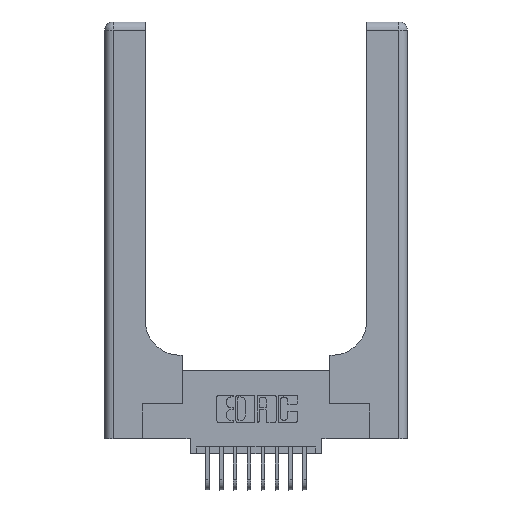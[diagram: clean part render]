
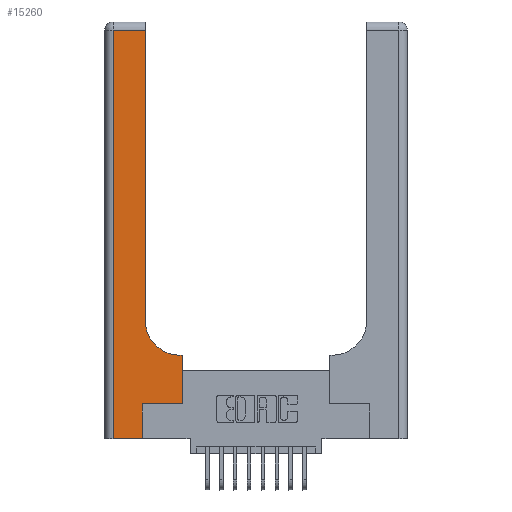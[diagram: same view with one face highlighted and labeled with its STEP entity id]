
A CAD part, top view. The second image highlights one B-rep face of the part: STEP entity #15260.
In plain terms, the highlighted planar face has unit normal (0, 0, 1).
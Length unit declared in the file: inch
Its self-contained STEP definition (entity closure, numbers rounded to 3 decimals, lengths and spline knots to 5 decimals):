
#75 = LINE ( 'NONE', #4057, #527 ) ;
#527 = VECTOR ( 'NONE', #12384, 39.37008 ) ;
#1086 = CARTESIAN_POINT ( 'NONE',  ( 0.2915, 2.94, 0.37 ) ) ;
#1235 = CARTESIAN_POINT ( 'NONE',  ( 0.2915, 0.6, 0.37 ) ) ;
#1479 = PLANE ( 'NONE',  #1958 ) ;
#1505 = CARTESIAN_POINT ( 'NONE',  ( 0.5415, 0.6, 0.37 ) ) ;
#1958 = AXIS2_PLACEMENT_3D ( 'NONE', #9866, #2883, #12638 ) ;
#2146 = CARTESIAN_POINT ( 'NONE',  ( 0.2915, 3., 0.37 ) ) ;
#2155 = VECTOR ( 'NONE', #7720, 39.37008 ) ;
#2588 = LINE ( 'NONE', #2146, #2155 ) ;
#2624 = CARTESIAN_POINT ( 'NONE',  ( 0.269, 0., 0.37 ) ) ;
#2649 = DIRECTION ( 'NONE',  ( -1., 0., 0. ) ) ;
#2883 = DIRECTION ( 'NONE',  ( 0., 0., -1. ) ) ;
#3165 = LINE ( 'NONE', #17815, #17306 ) ;
#3261 = VERTEX_POINT ( 'NONE', #2624 ) ;
#3745 = LINE ( 'NONE', #1235, #10744 ) ;
#3782 = ORIENTED_EDGE ( 'NONE', *, *, #10803, .T. ) ;
#3843 = EDGE_CURVE ( 'NONE', #6789, #8115, #2588, .T. ) ;
#4057 = CARTESIAN_POINT ( 'NONE',  ( 0.269, 0.25, 0.37 ) ) ;
#4095 = ORIENTED_EDGE ( 'NONE', *, *, #15156, .T. ) ;
#4213 = VECTOR ( 'NONE', #13894, 39.37008 ) ;
#4216 = VERTEX_POINT ( 'NONE', #5692 ) ;
#4262 = ORIENTED_EDGE ( 'NONE', *, *, #5912, .T. ) ;
#4640 = LINE ( 'NONE', #13652, #15166 ) ;
#4658 = LINE ( 'NONE', #5615, #4213 ) ;
#5382 = CIRCLE ( 'NONE', #16242, 0.25 ) ;
#5615 = CARTESIAN_POINT ( 'NONE',  ( 0.06, 3., 0.37 ) ) ;
#5692 = CARTESIAN_POINT ( 'NONE',  ( 0.06, 0., 0.37 ) ) ;
#5752 = CARTESIAN_POINT ( 'NONE',  ( 0.5415, 0.85, 0.37 ) ) ;
#5762 = EDGE_CURVE ( 'NONE', #10571, #16123, #75, .T. ) ;
#5819 = VECTOR ( 'NONE', #16554, 39.37008 ) ;
#5849 = EDGE_CURVE ( 'NONE', #4216, #3261, #11697, .T. ) ;
#5912 = EDGE_CURVE ( 'NONE', #14706, #6789, #5382, .T. ) ;
#6471 = EDGE_CURVE ( 'NONE', #8115, #14822, #3165, .T. ) ;
#6789 = VERTEX_POINT ( 'NONE', #10384 ) ;
#6978 = ORIENTED_EDGE ( 'NONE', *, *, #3843, .T. ) ;
#7153 = DIRECTION ( 'NONE',  ( 1., 0., 0. ) ) ;
#7691 = ORIENTED_EDGE ( 'NONE', *, *, #14671, .T. ) ;
#7720 = DIRECTION ( 'NONE',  ( 0., 1., 0. ) ) ;
#7810 = VECTOR ( 'NONE', #10729, 39.37008 ) ;
#8115 = VERTEX_POINT ( 'NONE', #1086 ) ;
#8242 = LINE ( 'NONE', #17394, #7810 ) ;
#8479 = VERTEX_POINT ( 'NONE', #12907 ) ;
#8580 = ORIENTED_EDGE ( 'NONE', *, *, #5762, .T. ) ;
#8990 = FACE_OUTER_BOUND ( 'NONE', #13356, .T. ) ;
#9780 = DIRECTION ( 'NONE',  ( -1., 0., 0. ) ) ;
#9866 = CARTESIAN_POINT ( 'NONE',  ( 0., 3., 0.37 ) ) ;
#10266 = CARTESIAN_POINT ( 'NONE',  ( 0.06, 2.94, 0.37 ) ) ;
#10384 = CARTESIAN_POINT ( 'NONE',  ( 0.2915, 0.85, 0.37 ) ) ;
#10571 = VERTEX_POINT ( 'NONE', #15611 ) ;
#10729 = DIRECTION ( 'NONE',  ( 0., 1., 0. ) ) ;
#10744 = VECTOR ( 'NONE', #2649, 39.37008 ) ;
#10803 = EDGE_CURVE ( 'NONE', #16123, #8479, #8242, .T. ) ;
#11697 = LINE ( 'NONE', #17825, #5819 ) ;
#12384 = DIRECTION ( 'NONE',  ( 1., 0., 0. ) ) ;
#12638 = DIRECTION ( 'NONE',  ( -1., 0., 0. ) ) ;
#12907 = CARTESIAN_POINT ( 'NONE',  ( 0.5585, 0.6, 0.37 ) ) ;
#13356 = EDGE_LOOP ( 'NONE', ( #6978, #17021, #7691, #13748, #15027, #8580, #3782, #4095, #4262 ) ) ;
#13652 = CARTESIAN_POINT ( 'NONE',  ( 0.269, 0., 0.37 ) ) ;
#13748 = ORIENTED_EDGE ( 'NONE', *, *, #5849, .T. ) ;
#13794 = CARTESIAN_POINT ( 'NONE',  ( 0.5585, 0.25, 0.37 ) ) ;
#13894 = DIRECTION ( 'NONE',  ( 0., -1., 0. ) ) ;
#14671 = EDGE_CURVE ( 'NONE', #14822, #4216, #4658, .T. ) ;
#14706 = VERTEX_POINT ( 'NONE', #1505 ) ;
#14822 = VERTEX_POINT ( 'NONE', #10266 ) ;
#15027 = ORIENTED_EDGE ( 'NONE', *, *, #15102, .T. ) ;
#15102 = EDGE_CURVE ( 'NONE', #3261, #10571, #4640, .T. ) ;
#15156 = EDGE_CURVE ( 'NONE', #8479, #14706, #3745, .T. ) ;
#15166 = VECTOR ( 'NONE', #17618, 39.37008 ) ;
#15260 = ADVANCED_FACE ( 'NONE', ( #8990 ), #1479, .F. ) ;
#15344 = DIRECTION ( 'NONE',  ( 0., 0., -1. ) ) ;
#15611 = CARTESIAN_POINT ( 'NONE',  ( 0.269, 0.25, 0.37 ) ) ;
#16123 = VERTEX_POINT ( 'NONE', #13794 ) ;
#16242 = AXIS2_PLACEMENT_3D ( 'NONE', #5752, #15344, #7153 ) ;
#16554 = DIRECTION ( 'NONE',  ( 1., 0., 0. ) ) ;
#17021 = ORIENTED_EDGE ( 'NONE', *, *, #6471, .T. ) ;
#17306 = VECTOR ( 'NONE', #9780, 39.37008 ) ;
#17394 = CARTESIAN_POINT ( 'NONE',  ( 0.5585, 0.25, 0.37 ) ) ;
#17618 = DIRECTION ( 'NONE',  ( 0., 1., 0. ) ) ;
#17815 = CARTESIAN_POINT ( 'NONE',  ( 0., 2.94, 0.37 ) ) ;
#17825 = CARTESIAN_POINT ( 'NONE',  ( 0., 0., 0.37 ) ) ;
